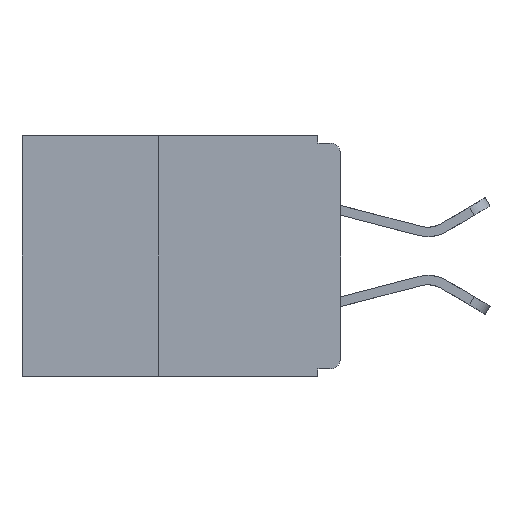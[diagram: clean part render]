
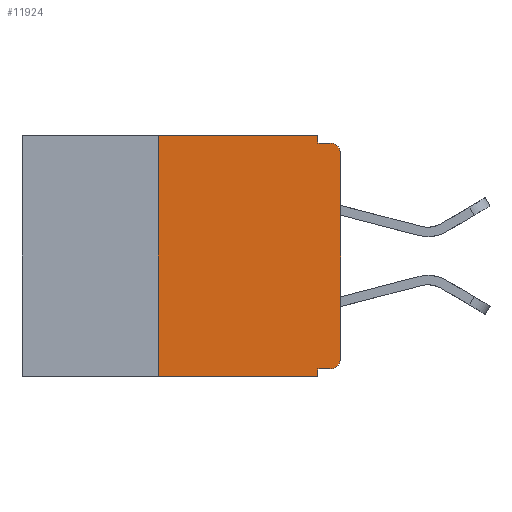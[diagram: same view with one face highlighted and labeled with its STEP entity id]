
A CAD part, left-side view. The second image highlights one B-rep face of the part: STEP entity #11924.
In plain terms, the highlighted planar face has unit normal (-1, 0, 0).
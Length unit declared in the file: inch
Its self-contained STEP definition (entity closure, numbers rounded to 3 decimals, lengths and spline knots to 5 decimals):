
#153 = CARTESIAN_POINT ( 'NONE',  ( 0., 0.25, -0.33 ) ) ;
#340 = DIRECTION ( 'NONE',  ( 0., 0., -1. ) ) ;
#355 = EDGE_CURVE ( 'NONE', #487, #9067, #12485, .T. ) ;
#487 = VERTEX_POINT ( 'NONE', #12949 ) ;
#793 = ORIENTED_EDGE ( 'NONE', *, *, #355, .F. ) ;
#837 = CARTESIAN_POINT ( 'NONE',  ( 0., 0.031, -0.33 ) ) ;
#1008 = ORIENTED_EDGE ( 'NONE', *, *, #9132, .T. ) ;
#1123 = CARTESIAN_POINT ( 'NONE',  ( 0., 0.031, -0.32 ) ) ;
#1270 = DIRECTION ( 'NONE',  ( 0., 0., 1. ) ) ;
#1282 = VERTEX_POINT ( 'NONE', #11983 ) ;
#1713 = CARTESIAN_POINT ( 'NONE',  ( 0., 0.437, 0. ) ) ;
#1726 = VERTEX_POINT ( 'NONE', #5547 ) ;
#1869 = CARTESIAN_POINT ( 'NONE',  ( 0., 0.437, 0. ) ) ;
#2630 = LINE ( 'NONE', #1713, #11642 ) ;
#2933 = VERTEX_POINT ( 'NONE', #1123 ) ;
#3571 = CARTESIAN_POINT ( 'NONE',  ( 0., 0., 0. ) ) ;
#4026 = DIRECTION ( 'NONE',  ( 0., -1., 0. ) ) ;
#4214 = EDGE_CURVE ( 'NONE', #9067, #1726, #13056, .T. ) ;
#4647 = CARTESIAN_POINT ( 'NONE',  ( 0., 0.031, -0.01 ) ) ;
#5024 = VERTEX_POINT ( 'NONE', #12834 ) ;
#5303 = DIRECTION ( 'NONE',  ( 1., 0., 0. ) ) ;
#5366 = CARTESIAN_POINT ( 'NONE',  ( 0., 0.015, -0.025 ) ) ;
#5517 = VERTEX_POINT ( 'NONE', #11875 ) ;
#5547 = CARTESIAN_POINT ( 'NONE',  ( 0., 0.015, -0.01 ) ) ;
#5623 = AXIS2_PLACEMENT_3D ( 'NONE', #1869, #5303, #13133 ) ;
#5813 = DIRECTION ( 'NONE',  ( 0., -1., 0. ) ) ;
#5898 = CARTESIAN_POINT ( 'NONE',  ( 0., 0., -0.32 ) ) ;
#5992 = DIRECTION ( 'NONE',  ( 0., 0., -1. ) ) ;
#5995 = VECTOR ( 'NONE', #11654, 39.37008 ) ;
#6165 = VECTOR ( 'NONE', #5992, 39.37008 ) ;
#6306 = AXIS2_PLACEMENT_3D ( 'NONE', #5366, #13197, #6552 ) ;
#6552 = DIRECTION ( 'NONE',  ( 0., 0., -1. ) ) ;
#6641 = ORIENTED_EDGE ( 'NONE', *, *, #4214, .F. ) ;
#6668 = FACE_OUTER_BOUND ( 'NONE', #10921, .T. ) ;
#6811 = VECTOR ( 'NONE', #12154, 39.37008 ) ;
#7081 = VERTEX_POINT ( 'NONE', #12451 ) ;
#7258 = VERTEX_POINT ( 'NONE', #9493 ) ;
#7292 = CIRCLE ( 'NONE', #13857, 0.015 ) ;
#7331 = DIRECTION ( 'NONE',  ( -1., 0., 0. ) ) ;
#7649 = CARTESIAN_POINT ( 'NONE',  ( 0., 0., -0.025 ) ) ;
#7730 = ORIENTED_EDGE ( 'NONE', *, *, #14295, .F. ) ;
#8701 = VECTOR ( 'NONE', #1270, 39.37008 ) ;
#8712 = CARTESIAN_POINT ( 'NONE',  ( 0., 0.031, 0. ) ) ;
#8748 = PLANE ( 'NONE',  #5623 ) ;
#9067 = VERTEX_POINT ( 'NONE', #4647 ) ;
#9132 = EDGE_CURVE ( 'NONE', #5024, #7258, #7292, .T. ) ;
#9276 = CIRCLE ( 'NONE', #6306, 0.015 ) ;
#9328 = ORIENTED_EDGE ( 'NONE', *, *, #12791, .T. ) ;
#9373 = CARTESIAN_POINT ( 'NONE',  ( 0., 0., -0.01 ) ) ;
#9493 = CARTESIAN_POINT ( 'NONE',  ( 0., 0., -0.305 ) ) ;
#9968 = EDGE_CURVE ( 'NONE', #7081, #487, #2630, .T. ) ;
#10039 = ORIENTED_EDGE ( 'NONE', *, *, #9968, .F. ) ;
#10100 = DIRECTION ( 'NONE',  ( 0., 0., -1. ) ) ;
#10313 = VECTOR ( 'NONE', #5813, 39.37008 ) ;
#10355 = EDGE_CURVE ( 'NONE', #7258, #13323, #11972, .T. ) ;
#10707 = ORIENTED_EDGE ( 'NONE', *, *, #13580, .T. ) ;
#10921 = EDGE_LOOP ( 'NONE', ( #11893, #9328, #6641, #793, #10039, #7730, #10707, #13567, #12745, #1008 ) ) ;
#11170 = LINE ( 'NONE', #837, #11506 ) ;
#11391 = CARTESIAN_POINT ( 'NONE',  ( 0., 0.437, -0.33 ) ) ;
#11506 = VECTOR ( 'NONE', #10100, 39.37008 ) ;
#11642 = VECTOR ( 'NONE', #4026, 39.37008 ) ;
#11654 = DIRECTION ( 'NONE',  ( 0., 0., 1. ) ) ;
#11875 = CARTESIAN_POINT ( 'NONE',  ( 0., 0.25, -0.33 ) ) ;
#11893 = ORIENTED_EDGE ( 'NONE', *, *, #10355, .T. ) ;
#11924 = ADVANCED_FACE ( 'NONE', ( #6668 ), #8748, .F. ) ;
#11972 = LINE ( 'NONE', #3571, #8701 ) ;
#11975 = LINE ( 'NONE', #153, #5995 ) ;
#11983 = CARTESIAN_POINT ( 'NONE',  ( 0., 0.031, -0.33 ) ) ;
#12154 = DIRECTION ( 'NONE',  ( 0., -1., 0. ) ) ;
#12451 = CARTESIAN_POINT ( 'NONE',  ( 0., 0.25, 0. ) ) ;
#12485 = LINE ( 'NONE', #8712, #6165 ) ;
#12745 = ORIENTED_EDGE ( 'NONE', *, *, #14212, .F. ) ;
#12791 = EDGE_CURVE ( 'NONE', #13323, #1726, #9276, .T. ) ;
#12834 = CARTESIAN_POINT ( 'NONE',  ( 0., 0.015, -0.32 ) ) ;
#12867 = EDGE_CURVE ( 'NONE', #2933, #1282, #11170, .T. ) ;
#12949 = CARTESIAN_POINT ( 'NONE',  ( 0., 0.031, 0. ) ) ;
#13056 = LINE ( 'NONE', #9373, #6811 ) ;
#13133 = DIRECTION ( 'NONE',  ( 0., 0., -1. ) ) ;
#13197 = DIRECTION ( 'NONE',  ( -1., 0., 0. ) ) ;
#13309 = VECTOR ( 'NONE', #13673, 39.37008 ) ;
#13323 = VERTEX_POINT ( 'NONE', #7649 ) ;
#13495 = LINE ( 'NONE', #11391, #10313 ) ;
#13567 = ORIENTED_EDGE ( 'NONE', *, *, #12867, .F. ) ;
#13580 = EDGE_CURVE ( 'NONE', #5517, #1282, #13495, .T. ) ;
#13673 = DIRECTION ( 'NONE',  ( 0., 1., 0. ) ) ;
#13857 = AXIS2_PLACEMENT_3D ( 'NONE', #13913, #7331, #340 ) ;
#13913 = CARTESIAN_POINT ( 'NONE',  ( 0., 0.015, -0.305 ) ) ;
#14212 = EDGE_CURVE ( 'NONE', #5024, #2933, #14312, .T. ) ;
#14295 = EDGE_CURVE ( 'NONE', #5517, #7081, #11975, .T. ) ;
#14312 = LINE ( 'NONE', #5898, #13309 ) ;
